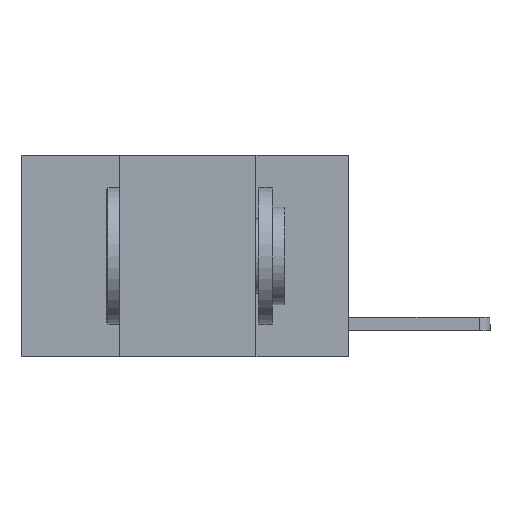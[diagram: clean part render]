
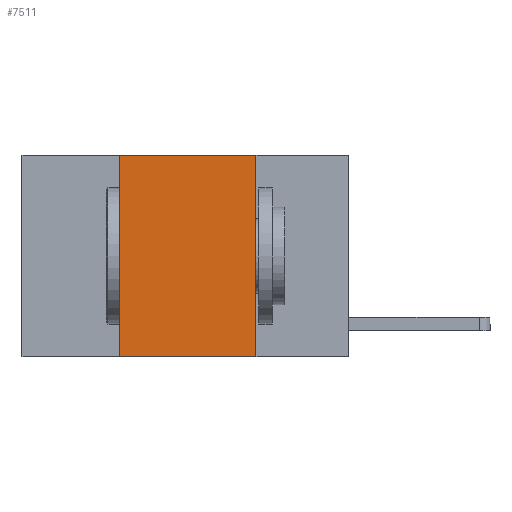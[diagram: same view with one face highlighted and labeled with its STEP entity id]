
A CAD part, left-side view. The second image highlights one B-rep face of the part: STEP entity #7511.
In plain terms, the highlighted planar face has unit normal (-1, 0, 0).
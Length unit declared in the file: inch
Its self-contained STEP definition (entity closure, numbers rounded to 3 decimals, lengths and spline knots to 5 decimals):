
#36 = VECTOR ( 'NONE', #6895, 39.37008 ) ;
#94 = EDGE_CURVE ( 'NONE', #6361, #7026, #8203, .T. ) ;
#425 = CARTESIAN_POINT ( 'NONE',  ( 0., 0.42, 0. ) ) ;
#754 = ORIENTED_EDGE ( 'NONE', *, *, #94, .F. ) ;
#787 = ORIENTED_EDGE ( 'NONE', *, *, #5699, .F. ) ;
#1096 = DIRECTION ( 'NONE',  ( 0., 0., 1. ) ) ;
#1464 = AXIS2_PLACEMENT_3D ( 'NONE', #1633, #2402, #4407 ) ;
#1633 = CARTESIAN_POINT ( 'NONE',  ( 0., 0.6, 0. ) ) ;
#1651 = ORIENTED_EDGE ( 'NONE', *, *, #2500, .T. ) ;
#1653 = DIRECTION ( 'NONE',  ( 0., -1., 0. ) ) ;
#2195 = EDGE_LOOP ( 'NONE', ( #5485, #754, #787, #1651 ) ) ;
#2299 = DIRECTION ( 'NONE',  ( 0., 0., -1. ) ) ;
#2402 = DIRECTION ( 'NONE',  ( 1., 0., 0. ) ) ;
#2411 = CARTESIAN_POINT ( 'NONE',  ( 0., 0.42, 0. ) ) ;
#2500 = EDGE_CURVE ( 'NONE', #8228, #7379, #3713, .T. ) ;
#2740 = CARTESIAN_POINT ( 'NONE',  ( 0., 0.42, -0.37 ) ) ;
#3279 = EDGE_CURVE ( 'NONE', #7026, #7379, #8512, .T. ) ;
#3713 = LINE ( 'NONE', #4913, #4868 ) ;
#4407 = DIRECTION ( 'NONE',  ( 0., 0., -1. ) ) ;
#4443 = CARTESIAN_POINT ( 'NONE',  ( 0., 0.17, 0. ) ) ;
#4801 = CARTESIAN_POINT ( 'NONE',  ( 0., 0.17, -0.37 ) ) ;
#4805 = CARTESIAN_POINT ( 'NONE',  ( 0., 0.6, 0. ) ) ;
#4868 = VECTOR ( 'NONE', #1653, 39.37008 ) ;
#4913 = CARTESIAN_POINT ( 'NONE',  ( 0., 0.6, -0.37 ) ) ;
#4940 = CARTESIAN_POINT ( 'NONE',  ( 0., 0.17, 0. ) ) ;
#5074 = LINE ( 'NONE', #2411, #7290 ) ;
#5159 = VECTOR ( 'NONE', #2299, 39.37008 ) ;
#5485 = ORIENTED_EDGE ( 'NONE', *, *, #3279, .F. ) ;
#5699 = EDGE_CURVE ( 'NONE', #8228, #6361, #5074, .T. ) ;
#6361 = VERTEX_POINT ( 'NONE', #425 ) ;
#6895 = DIRECTION ( 'NONE',  ( 0., -1., 0. ) ) ;
#7026 = VERTEX_POINT ( 'NONE', #4940 ) ;
#7290 = VECTOR ( 'NONE', #1096, 39.37008 ) ;
#7379 = VERTEX_POINT ( 'NONE', #4801 ) ;
#7511 = ADVANCED_FACE ( 'NONE', ( #7832 ), #8417, .F. ) ;
#7832 = FACE_OUTER_BOUND ( 'NONE', #2195, .T. ) ;
#8203 = LINE ( 'NONE', #4805, #36 ) ;
#8228 = VERTEX_POINT ( 'NONE', #2740 ) ;
#8417 = PLANE ( 'NONE',  #1464 ) ;
#8512 = LINE ( 'NONE', #4443, #5159 ) ;
